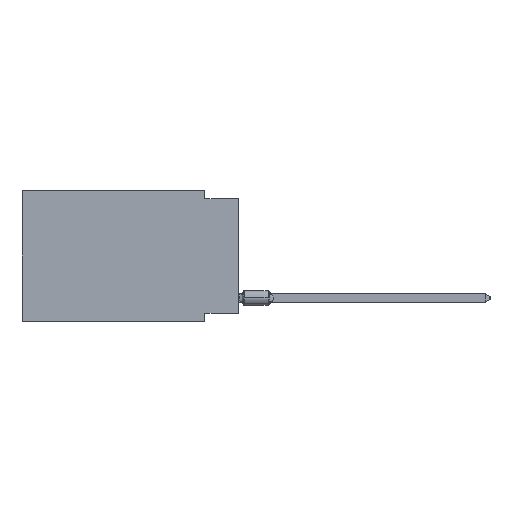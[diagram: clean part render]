
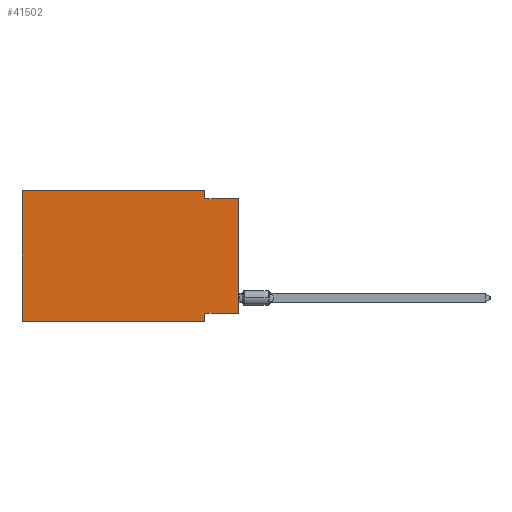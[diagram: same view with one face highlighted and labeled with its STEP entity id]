
A CAD part, left-side view. The second image highlights one B-rep face of the part: STEP entity #41502.
In plain terms, the highlighted planar face has unit normal (-1, 0, 0).
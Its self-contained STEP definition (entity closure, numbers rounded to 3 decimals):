
#724 = EDGE_CURVE ( 'NONE', #46533, #26008, #25534, .T. ) ;
#1294 = EDGE_CURVE ( 'NONE', #11334, #9115, #19877, .T. ) ;
#3093 = LINE ( 'NONE', #51687, #15267 ) ;
#3161 = LINE ( 'NONE', #44331, #42633 ) ;
#3246 = ORIENTED_EDGE ( 'NONE', *, *, #1294, .T. ) ;
#3912 = DIRECTION ( 'NONE',  ( 0., -1., 0. ) ) ;
#4259 = ORIENTED_EDGE ( 'NONE', *, *, #724, .F. ) ;
#4987 = VECTOR ( 'NONE', #3912, 1000. ) ;
#5330 = DIRECTION ( 'NONE',  ( 0., 0., -1. ) ) ;
#6219 = CARTESIAN_POINT ( 'NONE',  ( 0., 2.54, -9.271 ) ) ;
#6273 = EDGE_CURVE ( 'NONE', #48730, #46533, #8830, .T. ) ;
#6942 = EDGE_CURVE ( 'NONE', #27222, #48730, #3161, .T. ) ;
#8830 = LINE ( 'NONE', #25048, #36620 ) ;
#9115 = VERTEX_POINT ( 'NONE', #30513 ) ;
#9346 = DIRECTION ( 'NONE',  ( 0., 1., 0. ) ) ;
#9424 = LINE ( 'NONE', #25117, #21065 ) ;
#10121 = CARTESIAN_POINT ( 'NONE',  ( 0., 0., -0.635 ) ) ;
#11334 = VERTEX_POINT ( 'NONE', #41437 ) ;
#12327 = VERTEX_POINT ( 'NONE', #6219 ) ;
#12506 = PLANE ( 'NONE',  #14166 ) ;
#12648 = CARTESIAN_POINT ( 'NONE',  ( 0., 16.383, -9.906 ) ) ;
#13062 = DIRECTION ( 'NONE',  ( 0., 0., 1. ) ) ;
#13975 = VERTEX_POINT ( 'NONE', #27933 ) ;
#14166 = AXIS2_PLACEMENT_3D ( 'NONE', #48622, #29481, #5330 ) ;
#14803 = CARTESIAN_POINT ( 'NONE',  ( 0., 2.54, 0. ) ) ;
#15267 = VECTOR ( 'NONE', #47706, 1000. ) ;
#16743 = ORIENTED_EDGE ( 'NONE', *, *, #6942, .F. ) ;
#16954 = VECTOR ( 'NONE', #13062, 1000. ) ;
#18350 = EDGE_CURVE ( 'NONE', #13975, #12327, #29018, .T. ) ;
#18354 = ORIENTED_EDGE ( 'NONE', *, *, #43863, .F. ) ;
#19877 = LINE ( 'NONE', #12648, #4987 ) ;
#21065 = VECTOR ( 'NONE', #45802, 1000. ) ;
#21564 = DIRECTION ( 'NONE',  ( 0., -1., 0. ) ) ;
#21846 = CARTESIAN_POINT ( 'NONE',  ( 0., 0., -9.271 ) ) ;
#25037 = CARTESIAN_POINT ( 'NONE',  ( 0., 0., 0. ) ) ;
#25048 = CARTESIAN_POINT ( 'NONE',  ( 0., 2.54, 0. ) ) ;
#25117 = CARTESIAN_POINT ( 'NONE',  ( 0., 2.54, -9.906 ) ) ;
#25534 = LINE ( 'NONE', #10121, #50754 ) ;
#26008 = VERTEX_POINT ( 'NONE', #31641 ) ;
#27222 = VERTEX_POINT ( 'NONE', #30243 ) ;
#27933 = CARTESIAN_POINT ( 'NONE',  ( 0., 0., -9.271 ) ) ;
#29018 = LINE ( 'NONE', #21846, #47544 ) ;
#29481 = DIRECTION ( 'NONE',  ( 1., 0., 0. ) ) ;
#29871 = ORIENTED_EDGE ( 'NONE', *, *, #6273, .F. ) ;
#30243 = CARTESIAN_POINT ( 'NONE',  ( 0., 16.383, 0. ) ) ;
#30513 = CARTESIAN_POINT ( 'NONE',  ( 0., 2.54, -9.906 ) ) ;
#31641 = CARTESIAN_POINT ( 'NONE',  ( 0., 0., -0.635 ) ) ;
#32717 = CARTESIAN_POINT ( 'NONE',  ( 0., 2.54, -0.635 ) ) ;
#33717 = EDGE_LOOP ( 'NONE', ( #49220, #4259, #29871, #16743, #18354, #3246, #44061, #43295 ) ) ;
#35576 = DIRECTION ( 'NONE',  ( 0., -1., 0. ) ) ;
#36620 = VECTOR ( 'NONE', #41254, 1000. ) ;
#40625 = EDGE_CURVE ( 'NONE', #12327, #9115, #9424, .T. ) ;
#41254 = DIRECTION ( 'NONE',  ( 0., 0., -1. ) ) ;
#41437 = CARTESIAN_POINT ( 'NONE',  ( 0., 16.383, -9.906 ) ) ;
#41502 = ADVANCED_FACE ( 'NONE', ( #44651 ), #12506, .F. ) ;
#42633 = VECTOR ( 'NONE', #35576, 1000. ) ;
#43295 = ORIENTED_EDGE ( 'NONE', *, *, #18350, .F. ) ;
#43863 = EDGE_CURVE ( 'NONE', #11334, #27222, #3093, .T. ) ;
#43894 = EDGE_CURVE ( 'NONE', #13975, #26008, #49445, .T. ) ;
#44061 = ORIENTED_EDGE ( 'NONE', *, *, #40625, .F. ) ;
#44331 = CARTESIAN_POINT ( 'NONE',  ( 0., 16.383, 0. ) ) ;
#44651 = FACE_OUTER_BOUND ( 'NONE', #33717, .T. ) ;
#45802 = DIRECTION ( 'NONE',  ( 0., 0., -1. ) ) ;
#46533 = VERTEX_POINT ( 'NONE', #32717 ) ;
#47544 = VECTOR ( 'NONE', #9346, 1000. ) ;
#47706 = DIRECTION ( 'NONE',  ( 0., 0., 1. ) ) ;
#48622 = CARTESIAN_POINT ( 'NONE',  ( 0., 16.383, 0. ) ) ;
#48730 = VERTEX_POINT ( 'NONE', #14803 ) ;
#49220 = ORIENTED_EDGE ( 'NONE', *, *, #43894, .T. ) ;
#49445 = LINE ( 'NONE', #25037, #16954 ) ;
#50754 = VECTOR ( 'NONE', #21564, 1000. ) ;
#51687 = CARTESIAN_POINT ( 'NONE',  ( 0., 16.383, 0. ) ) ;
